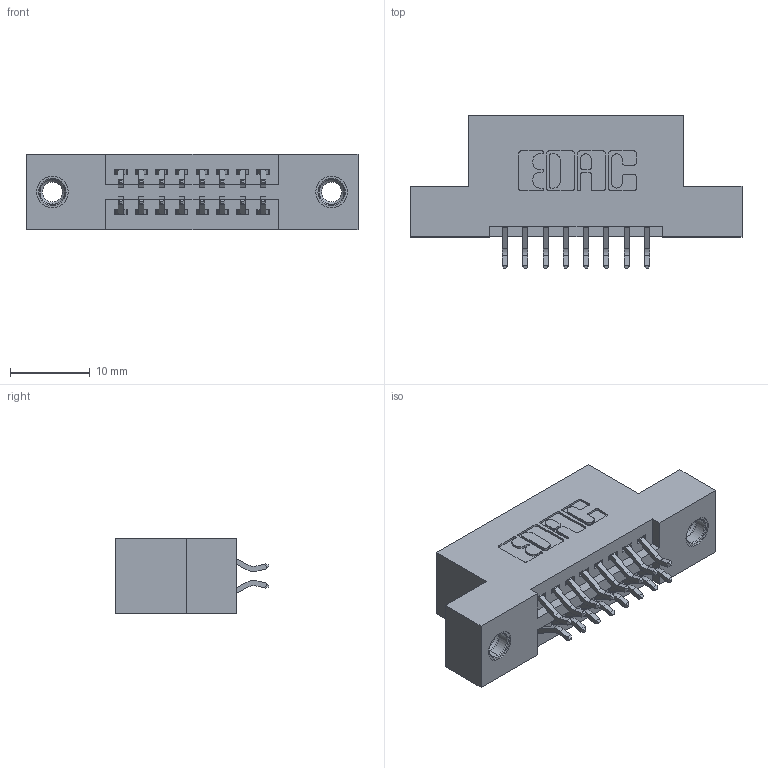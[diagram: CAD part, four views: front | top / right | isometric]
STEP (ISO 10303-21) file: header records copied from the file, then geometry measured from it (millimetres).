
FILE_DESCRIPTION (( 'STEP AP203' ), '1' );
FILE_NAME ('345-016-556-207.STEP', '2019-10-27T04:47:09', ( '' ), ( '' ), 'SwSTEP 2.0', 'SolidWorks 2016', '' );
FILE_SCHEMA (( 'CONFIG_CONTROL_DESIGN' ));
Length unit declared in the file: inch
Products named in the file (4): 345-292-001_556 Tail; 345 Part_Flush Mounting Lugs - 0.156 Dia-TI; 345-016-556-207; 345-250-001_345-250-005-103
Assembly tree (19 placements, depth 2):
  345-016-556-207
    345 Part_Flush Mounting Lugs - 0.156 Dia-TI
    345-292-001_556 Tail  x16
    345-250-001_345-250-005-103  x2
Bounding box: 41.53 x 19.24 x 9.4 mm (x, y, z)
Volume: 3704.4 mm3; surface area: 4831.1 mm2
Topology: 19 solids, 19 shells, 1082 faces, 3149 edges, 2070 vertices
Faces by surface type: plane 704, cylinder 362, cone 12, torus 4
Entity records: 12260 total; most frequent: CARTESIAN_POINT 2083, ORIENTED_EDGE 1998, DIRECTION 1893, EDGE_CURVE 999, LINE 807, VECTOR 807, VERTEX_POINT 660, AXIS2_PLACEMENT_3D 543
